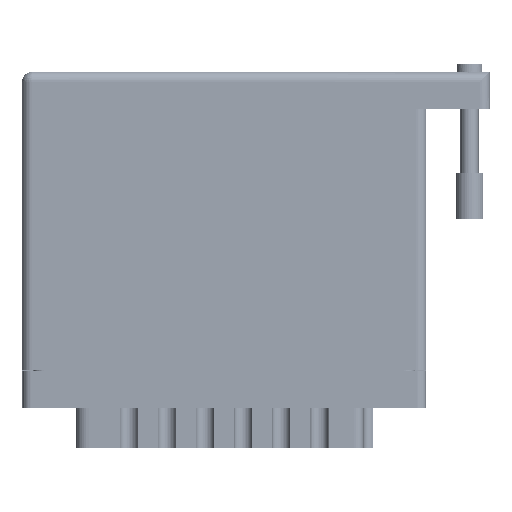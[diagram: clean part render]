
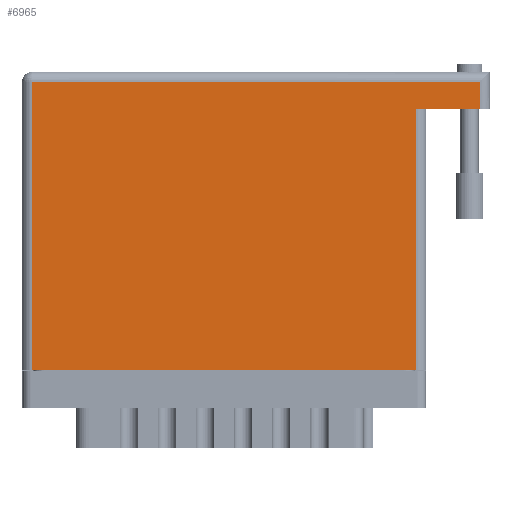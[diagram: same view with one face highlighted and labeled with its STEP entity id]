
A CAD part, front view. The second image highlights one B-rep face of the part: STEP entity #6965.
In plain terms, the highlighted face is planar.
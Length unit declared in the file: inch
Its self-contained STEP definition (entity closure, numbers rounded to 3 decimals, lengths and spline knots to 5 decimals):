
#1673 = DIRECTION ( 'NONE',  ( -1., 0., 0. ) ) ;
#2547 = EDGE_LOOP ( 'NONE', ( #36366, #10776, #40780, #8354, #72489, #78764 ) ) ;
#2572 = LINE ( 'NONE', #91338, #57329 ) ;
#3840 = PLANE ( 'NONE',  #13297 ) ;
#6965 = ADVANCED_FACE ( 'NONE', ( #19464 ), #3840, .F. ) ;
#7614 = CARTESIAN_POINT ( 'NONE',  ( 0.07, 1.96, 0. ) ) ;
#8354 = ORIENTED_EDGE ( 'NONE', *, *, #21429, .T. ) ;
#8690 = VECTOR ( 'NONE', #48578, 39.37008 ) ;
#10776 = ORIENTED_EDGE ( 'NONE', *, *, #29598, .T. ) ;
#11340 = VECTOR ( 'NONE', #1673, 39.37008 ) ;
#12461 = DIRECTION ( 'NONE',  ( 0., -1., 0. ) ) ;
#12582 = VERTEX_POINT ( 'NONE', #92154 ) ;
#13037 = LINE ( 'NONE', #35702, #49100 ) ;
#13297 = AXIS2_PLACEMENT_3D ( 'NONE', #84937, #55605, #18267 ) ;
#16648 = CARTESIAN_POINT ( 'NONE',  ( 2.685, 0., 0. ) ) ;
#18267 = DIRECTION ( 'NONE',  ( -1., 0., 0. ) ) ;
#18995 = CARTESIAN_POINT ( 'NONE',  ( 0.07, 0., 0. ) ) ;
#19464 = FACE_OUTER_BOUND ( 'NONE', #2547, .T. ) ;
#19959 = VECTOR ( 'NONE', #27585, 39.37008 ) ;
#20163 = EDGE_CURVE ( 'NONE', #25745, #30975, #35433, .T. ) ;
#21429 = EDGE_CURVE ( 'NONE', #81033, #12582, #2572, .T. ) ;
#23691 = VERTEX_POINT ( 'NONE', #7614 ) ;
#24616 = LINE ( 'NONE', #34691, #19959 ) ;
#25745 = VERTEX_POINT ( 'NONE', #18995 ) ;
#27100 = CARTESIAN_POINT ( 'NONE',  ( 0.07, 0., 0. ) ) ;
#27585 = DIRECTION ( 'NONE',  ( -1., 0., 0. ) ) ;
#29598 = EDGE_CURVE ( 'NONE', #30975, #32935, #13037, .T. ) ;
#30975 = VERTEX_POINT ( 'NONE', #16648 ) ;
#31115 = LINE ( 'NONE', #76273, #11340 ) ;
#32935 = VERTEX_POINT ( 'NONE', #78698 ) ;
#34691 = CARTESIAN_POINT ( 'NONE',  ( 0., 1.96, 0. ) ) ;
#35433 = LINE ( 'NONE', #56097, #8690 ) ;
#35702 = CARTESIAN_POINT ( 'NONE',  ( 2.685, 1.774, 0. ) ) ;
#36366 = ORIENTED_EDGE ( 'NONE', *, *, #20163, .T. ) ;
#39488 = LINE ( 'NONE', #27100, #42941 ) ;
#40780 = ORIENTED_EDGE ( 'NONE', *, *, #85853, .F. ) ;
#41589 = EDGE_CURVE ( 'NONE', #23691, #25745, #39488, .T. ) ;
#42941 = VECTOR ( 'NONE', #12461, 39.37008 ) ;
#46184 = EDGE_CURVE ( 'NONE', #12582, #23691, #24616, .T. ) ;
#48578 = DIRECTION ( 'NONE',  ( 1., 0., 0. ) ) ;
#49100 = VECTOR ( 'NONE', #87506, 39.37008 ) ;
#55605 = DIRECTION ( 'NONE',  ( 0., 0., -1. ) ) ;
#56097 = CARTESIAN_POINT ( 'NONE',  ( 0., 0., 0. ) ) ;
#57329 = VECTOR ( 'NONE', #76068, 39.37008 ) ;
#72489 = ORIENTED_EDGE ( 'NONE', *, *, #46184, .T. ) ;
#76068 = DIRECTION ( 'NONE',  ( 0., 1., 0. ) ) ;
#76273 = CARTESIAN_POINT ( 'NONE',  ( 3.19, 1.774, 0. ) ) ;
#76837 = CARTESIAN_POINT ( 'NONE',  ( 3.12, 1.774, 0. ) ) ;
#78698 = CARTESIAN_POINT ( 'NONE',  ( 2.685, 1.774, 0. ) ) ;
#78764 = ORIENTED_EDGE ( 'NONE', *, *, #41589, .T. ) ;
#81033 = VERTEX_POINT ( 'NONE', #76837 ) ;
#84937 = CARTESIAN_POINT ( 'NONE',  ( 0., 2.03, 0. ) ) ;
#85853 = EDGE_CURVE ( 'NONE', #81033, #32935, #31115, .T. ) ;
#87506 = DIRECTION ( 'NONE',  ( 0., 1., 0. ) ) ;
#91338 = CARTESIAN_POINT ( 'NONE',  ( 3.12, 2.03, 0. ) ) ;
#92154 = CARTESIAN_POINT ( 'NONE',  ( 3.12, 1.96, 0. ) ) ;
